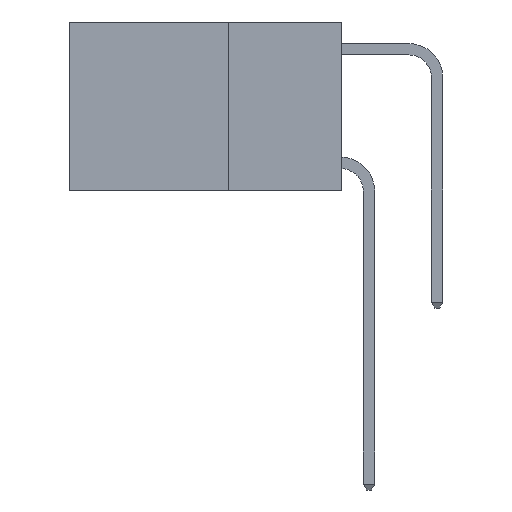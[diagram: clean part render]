
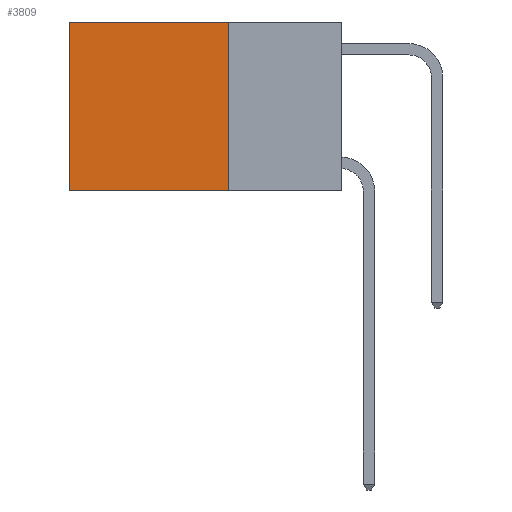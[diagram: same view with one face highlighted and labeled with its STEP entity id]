
A CAD part, left-side view. The second image highlights one B-rep face of the part: STEP entity #3809.
In plain terms, the highlighted planar face has unit normal (-1, 0, 0).
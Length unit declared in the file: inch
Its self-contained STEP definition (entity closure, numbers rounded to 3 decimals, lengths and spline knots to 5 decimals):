
#145 = EDGE_CURVE ( 'NONE', #7950, #1975, #8301, .T. ) ;
#560 = CARTESIAN_POINT ( 'NONE',  ( 0.2625, 0.6, 0. ) ) ;
#673 = EDGE_CURVE ( 'NONE', #6891, #7950, #13316, .T. ) ;
#1089 = EDGE_LOOP ( 'NONE', ( #6219, #12997, #6073, #12421 ) ) ;
#1101 = CARTESIAN_POINT ( 'NONE',  ( 0.2625, 0.25, -0.37 ) ) ;
#1211 = AXIS2_PLACEMENT_3D ( 'NONE', #9151, #12303, #6000 ) ;
#1463 = CARTESIAN_POINT ( 'NONE',  ( 0.2625, 0.6, 0. ) ) ;
#1975 = VERTEX_POINT ( 'NONE', #10493 ) ;
#2703 = CARTESIAN_POINT ( 'NONE',  ( 0.2625, 0.25, -0.37 ) ) ;
#2884 = PLANE ( 'NONE',  #1211 ) ;
#3735 = DIRECTION ( 'NONE',  ( 0., 1., 0. ) ) ;
#3809 = ADVANCED_FACE ( 'NONE', ( #11800 ), #2884, .F. ) ;
#3841 = LINE ( 'NONE', #11786, #9101 ) ;
#4479 = VECTOR ( 'NONE', #3735, 39.37008 ) ;
#5460 = DIRECTION ( 'NONE',  ( 0., 0., -1. ) ) ;
#5617 = EDGE_CURVE ( 'NONE', #11287, #1975, #7330, .T. ) ;
#6000 = DIRECTION ( 'NONE',  ( 0., 0., -1. ) ) ;
#6073 = ORIENTED_EDGE ( 'NONE', *, *, #9668, .F. ) ;
#6219 = ORIENTED_EDGE ( 'NONE', *, *, #145, .T. ) ;
#6891 = VERTEX_POINT ( 'NONE', #9862 ) ;
#7330 = LINE ( 'NONE', #2703, #4479 ) ;
#7950 = VERTEX_POINT ( 'NONE', #1463 ) ;
#8301 = LINE ( 'NONE', #560, #11100 ) ;
#9101 = VECTOR ( 'NONE', #5460, 39.37008 ) ;
#9151 = CARTESIAN_POINT ( 'NONE',  ( 0.2625, 0.25, 0. ) ) ;
#9668 = EDGE_CURVE ( 'NONE', #6891, #11287, #3841, .T. ) ;
#9862 = CARTESIAN_POINT ( 'NONE',  ( 0.2625, 0.25, 0. ) ) ;
#10032 = DIRECTION ( 'NONE',  ( 0., 1., 0. ) ) ;
#10493 = CARTESIAN_POINT ( 'NONE',  ( 0.2625, 0.6, -0.37 ) ) ;
#10581 = VECTOR ( 'NONE', #10032, 39.37008 ) ;
#11095 = CARTESIAN_POINT ( 'NONE',  ( 0.2625, 0.25, 0. ) ) ;
#11100 = VECTOR ( 'NONE', #12048, 39.37008 ) ;
#11287 = VERTEX_POINT ( 'NONE', #1101 ) ;
#11786 = CARTESIAN_POINT ( 'NONE',  ( 0.2625, 0.25, 0. ) ) ;
#11800 = FACE_OUTER_BOUND ( 'NONE', #1089, .T. ) ;
#12048 = DIRECTION ( 'NONE',  ( 0., 0., -1. ) ) ;
#12303 = DIRECTION ( 'NONE',  ( 1., 0., 0. ) ) ;
#12421 = ORIENTED_EDGE ( 'NONE', *, *, #673, .T. ) ;
#12997 = ORIENTED_EDGE ( 'NONE', *, *, #5617, .F. ) ;
#13316 = LINE ( 'NONE', #11095, #10581 ) ;
